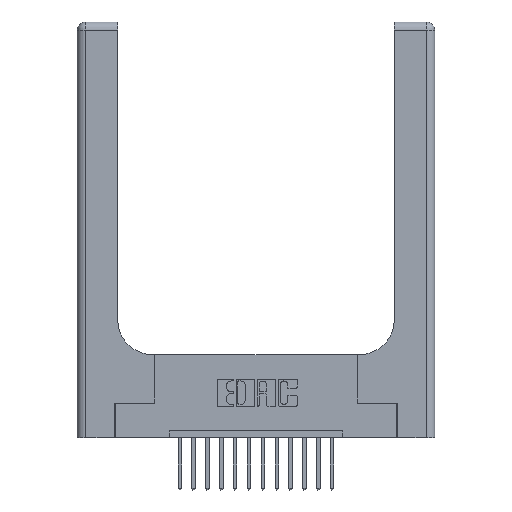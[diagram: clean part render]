
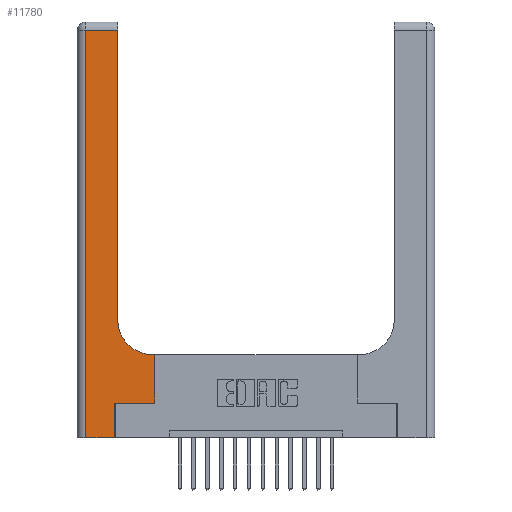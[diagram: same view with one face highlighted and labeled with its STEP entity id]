
A CAD part, top view. The second image highlights one B-rep face of the part: STEP entity #11780.
In plain terms, the highlighted planar face has unit normal (0, 0, 1).
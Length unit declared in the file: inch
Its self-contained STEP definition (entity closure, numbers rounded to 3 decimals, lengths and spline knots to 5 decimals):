
#455 = DIRECTION ( 'NONE',  ( 0., 0., -1. ) ) ;
#556 = EDGE_CURVE ( 'NONE', #744, #1238, #7819, .T. ) ;
#581 = DIRECTION ( 'NONE',  ( 1., 0., 0. ) ) ;
#744 = VERTEX_POINT ( 'NONE', #1720 ) ;
#953 = EDGE_CURVE ( 'NONE', #5502, #14299, #15740, .T. ) ;
#1130 = DIRECTION ( 'NONE',  ( -1., 0., 0. ) ) ;
#1191 = VERTEX_POINT ( 'NONE', #1968 ) ;
#1234 = PLANE ( 'NONE',  #3016 ) ;
#1238 = VERTEX_POINT ( 'NONE', #5782 ) ;
#1262 = VECTOR ( 'NONE', #3425, 39.37008 ) ;
#1720 = CARTESIAN_POINT ( 'NONE',  ( 0.269, 0.25, 0.37 ) ) ;
#1968 = CARTESIAN_POINT ( 'NONE',  ( 0.5415, 0.6, 0.37 ) ) ;
#2132 = CARTESIAN_POINT ( 'NONE',  ( 0.2915, 0.6, 0.37 ) ) ;
#2145 = CARTESIAN_POINT ( 'NONE',  ( 0.269, 0.25, 0.37 ) ) ;
#3016 = AXIS2_PLACEMENT_3D ( 'NONE', #4205, #5390, #4147 ) ;
#3326 = LINE ( 'NONE', #11157, #14778 ) ;
#3425 = DIRECTION ( 'NONE',  ( -1., 0., 0. ) ) ;
#3437 = VECTOR ( 'NONE', #14558, 39.37008 ) ;
#3492 = DIRECTION ( 'NONE',  ( 1., 0., 0. ) ) ;
#3585 = VECTOR ( 'NONE', #17001, 39.37008 ) ;
#3624 = CARTESIAN_POINT ( 'NONE',  ( 0.2915, 2.94, 0.37 ) ) ;
#3797 = LINE ( 'NONE', #10798, #14125 ) ;
#3878 = VERTEX_POINT ( 'NONE', #14845 ) ;
#3894 = AXIS2_PLACEMENT_3D ( 'NONE', #6076, #455, #581 ) ;
#4147 = DIRECTION ( 'NONE',  ( -1., 0., 0. ) ) ;
#4205 = CARTESIAN_POINT ( 'NONE',  ( 0., 3., 0.37 ) ) ;
#4742 = CARTESIAN_POINT ( 'NONE',  ( 0.5585, 0.25, 0.37 ) ) ;
#5203 = LINE ( 'NONE', #4742, #3437 ) ;
#5390 = DIRECTION ( 'NONE',  ( 0., 0., -1. ) ) ;
#5502 = VERTEX_POINT ( 'NONE', #5511 ) ;
#5511 = CARTESIAN_POINT ( 'NONE',  ( 0.2915, 0.85, 0.37 ) ) ;
#5782 = CARTESIAN_POINT ( 'NONE',  ( 0.5585, 0.25, 0.37 ) ) ;
#6076 = CARTESIAN_POINT ( 'NONE',  ( 0.5415, 0.85, 0.37 ) ) ;
#6415 = ORIENTED_EDGE ( 'NONE', *, *, #953, .T. ) ;
#6450 = ORIENTED_EDGE ( 'NONE', *, *, #9273, .T. ) ;
#6629 = VERTEX_POINT ( 'NONE', #7895 ) ;
#6713 = EDGE_CURVE ( 'NONE', #14299, #3878, #3326, .T. ) ;
#6816 = ORIENTED_EDGE ( 'NONE', *, *, #18174, .T. ) ;
#7272 = VERTEX_POINT ( 'NONE', #9221 ) ;
#7783 = FACE_OUTER_BOUND ( 'NONE', #9026, .T. ) ;
#7819 = LINE ( 'NONE', #2145, #16423 ) ;
#7895 = CARTESIAN_POINT ( 'NONE',  ( 0.5585, 0.6, 0.37 ) ) ;
#8390 = EDGE_CURVE ( 'NONE', #3878, #7272, #16046, .T. ) ;
#8508 = DIRECTION ( 'NONE',  ( 0., -1., 0. ) ) ;
#8562 = CARTESIAN_POINT ( 'NONE',  ( 0.06, 3., 0.37 ) ) ;
#8602 = CARTESIAN_POINT ( 'NONE',  ( 0.269, 0., 0.37 ) ) ;
#8760 = LINE ( 'NONE', #2132, #1262 ) ;
#9026 = EDGE_LOOP ( 'NONE', ( #6415, #11959, #10550, #6816, #11106, #9292, #15720, #6450, #10580 ) ) ;
#9221 = CARTESIAN_POINT ( 'NONE',  ( 0.06, 0., 0.37 ) ) ;
#9273 = EDGE_CURVE ( 'NONE', #6629, #1191, #8760, .T. ) ;
#9292 = ORIENTED_EDGE ( 'NONE', *, *, #556, .T. ) ;
#10108 = VECTOR ( 'NONE', #8508, 39.37008 ) ;
#10550 = ORIENTED_EDGE ( 'NONE', *, *, #8390, .T. ) ;
#10580 = ORIENTED_EDGE ( 'NONE', *, *, #14747, .T. ) ;
#10670 = EDGE_CURVE ( 'NONE', #1238, #6629, #5203, .T. ) ;
#10798 = CARTESIAN_POINT ( 'NONE',  ( 0., 0., 0.37 ) ) ;
#11049 = CIRCLE ( 'NONE', #3894, 0.25 ) ;
#11106 = ORIENTED_EDGE ( 'NONE', *, *, #17847, .T. ) ;
#11157 = CARTESIAN_POINT ( 'NONE',  ( 0., 2.94, 0.37 ) ) ;
#11780 = ADVANCED_FACE ( 'NONE', ( #7783 ), #1234, .F. ) ;
#11959 = ORIENTED_EDGE ( 'NONE', *, *, #6713, .T. ) ;
#12333 = CARTESIAN_POINT ( 'NONE',  ( 0.2915, 3., 0.37 ) ) ;
#14125 = VECTOR ( 'NONE', #14829, 39.37008 ) ;
#14195 = VECTOR ( 'NONE', #17753, 39.37008 ) ;
#14299 = VERTEX_POINT ( 'NONE', #3624 ) ;
#14361 = LINE ( 'NONE', #8602, #3585 ) ;
#14558 = DIRECTION ( 'NONE',  ( 0., 1., 0. ) ) ;
#14624 = CARTESIAN_POINT ( 'NONE',  ( 0.269, 0., 0.37 ) ) ;
#14747 = EDGE_CURVE ( 'NONE', #1191, #5502, #11049, .T. ) ;
#14778 = VECTOR ( 'NONE', #1130, 39.37008 ) ;
#14829 = DIRECTION ( 'NONE',  ( 1., 0., 0. ) ) ;
#14845 = CARTESIAN_POINT ( 'NONE',  ( 0.06, 2.94, 0.37 ) ) ;
#14850 = VERTEX_POINT ( 'NONE', #14624 ) ;
#15720 = ORIENTED_EDGE ( 'NONE', *, *, #10670, .T. ) ;
#15740 = LINE ( 'NONE', #12333, #14195 ) ;
#16046 = LINE ( 'NONE', #8562, #10108 ) ;
#16423 = VECTOR ( 'NONE', #3492, 39.37008 ) ;
#17001 = DIRECTION ( 'NONE',  ( 0., 1., 0. ) ) ;
#17753 = DIRECTION ( 'NONE',  ( 0., 1., 0. ) ) ;
#17847 = EDGE_CURVE ( 'NONE', #14850, #744, #14361, .T. ) ;
#18174 = EDGE_CURVE ( 'NONE', #7272, #14850, #3797, .T. ) ;
